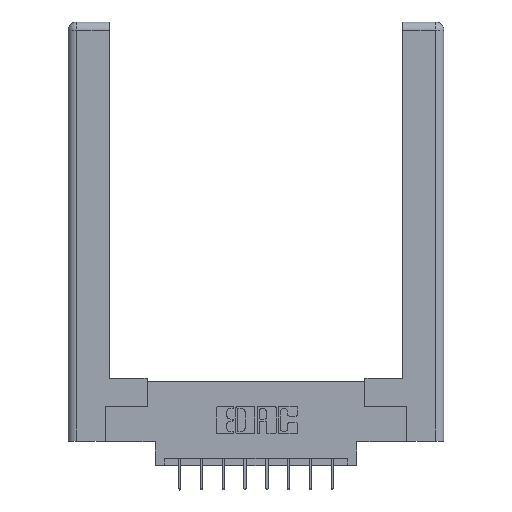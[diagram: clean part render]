
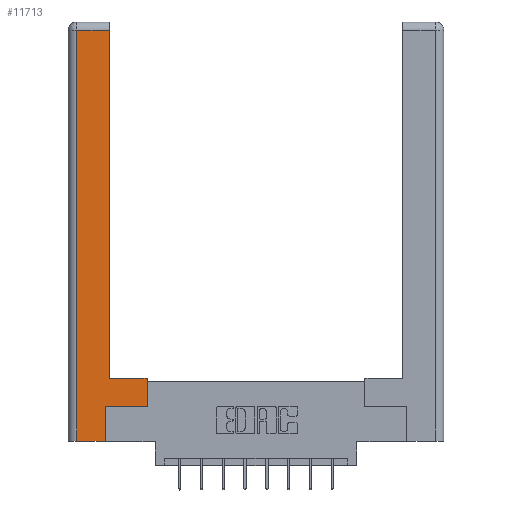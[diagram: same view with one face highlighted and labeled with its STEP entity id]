
A CAD part, top view. The second image highlights one B-rep face of the part: STEP entity #11713.
In plain terms, the highlighted planar face has unit normal (0, 0, 1).
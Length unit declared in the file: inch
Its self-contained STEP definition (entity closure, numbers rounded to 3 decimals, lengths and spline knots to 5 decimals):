
#439 = VERTEX_POINT ( 'NONE', #5067 ) ;
#670 = AXIS2_PLACEMENT_3D ( 'NONE', #10970, #13184, #11152 ) ;
#1038 = CARTESIAN_POINT ( 'NONE',  ( 0.265, 0.245, 0. ) ) ;
#1126 = DIRECTION ( 'NONE',  ( 0., 1., 0. ) ) ;
#1626 = LINE ( 'NONE', #8854, #5019 ) ;
#1725 = ORIENTED_EDGE ( 'NONE', *, *, #13055, .T. ) ;
#1729 = ORIENTED_EDGE ( 'NONE', *, *, #2698, .T. ) ;
#1742 = DIRECTION ( 'NONE',  ( -1., 0., 0. ) ) ;
#1770 = VECTOR ( 'NONE', #6748, 39.37008 ) ;
#1803 = CARTESIAN_POINT ( 'NONE',  ( 0.265, 0., 0. ) ) ;
#1998 = DIRECTION ( 'NONE',  ( 1., 0., 0. ) ) ;
#2093 = EDGE_CURVE ( 'NONE', #8377, #6248, #12899, .T. ) ;
#2221 = VERTEX_POINT ( 'NONE', #5303 ) ;
#2244 = CARTESIAN_POINT ( 'NONE',  ( 0.295, 0.45, 0. ) ) ;
#2698 = EDGE_CURVE ( 'NONE', #7606, #6331, #7299, .T. ) ;
#3141 = EDGE_CURVE ( 'NONE', #6331, #7619, #6506, .T. ) ;
#3749 = ORIENTED_EDGE ( 'NONE', *, *, #11745, .T. ) ;
#4716 = CARTESIAN_POINT ( 'NONE',  ( 0.295, 3., 0. ) ) ;
#4830 = CARTESIAN_POINT ( 'NONE',  ( 0.565, 0.245, 0. ) ) ;
#5000 = CARTESIAN_POINT ( 'NONE',  ( 0.0615, 0., 0. ) ) ;
#5019 = VECTOR ( 'NONE', #1742, 39.37008 ) ;
#5067 = CARTESIAN_POINT ( 'NONE',  ( 0.565, 0.45, 0. ) ) ;
#5303 = CARTESIAN_POINT ( 'NONE',  ( 0.295, 2.94, 0. ) ) ;
#5574 = ORIENTED_EDGE ( 'NONE', *, *, #13428, .T. ) ;
#5677 = FACE_OUTER_BOUND ( 'NONE', #7640, .T. ) ;
#6065 = CARTESIAN_POINT ( 'NONE',  ( 0.565, 0.245, 0. ) ) ;
#6248 = VERTEX_POINT ( 'NONE', #4830 ) ;
#6330 = DIRECTION ( 'NONE',  ( 0., 1., 0. ) ) ;
#6331 = VERTEX_POINT ( 'NONE', #5000 ) ;
#6367 = ORIENTED_EDGE ( 'NONE', *, *, #8719, .T. ) ;
#6506 = LINE ( 'NONE', #10055, #7625 ) ;
#6741 = ORIENTED_EDGE ( 'NONE', *, *, #3141, .T. ) ;
#6748 = DIRECTION ( 'NONE',  ( 0., 1., 0. ) ) ;
#7018 = DIRECTION ( 'NONE',  ( -1., 0., 0. ) ) ;
#7156 = EDGE_CURVE ( 'NONE', #6248, #439, #10647, .T. ) ;
#7299 = LINE ( 'NONE', #7447, #9768 ) ;
#7447 = CARTESIAN_POINT ( 'NONE',  ( 0.0615, 0., 0. ) ) ;
#7606 = VERTEX_POINT ( 'NONE', #7853 ) ;
#7619 = VERTEX_POINT ( 'NONE', #1803 ) ;
#7625 = VECTOR ( 'NONE', #9105, 39.37008 ) ;
#7640 = EDGE_LOOP ( 'NONE', ( #1725, #3749, #1729, #6741, #5574, #8189, #9995, #6367 ) ) ;
#7853 = CARTESIAN_POINT ( 'NONE',  ( 0.0615, 2.94, 0. ) ) ;
#7855 = VECTOR ( 'NONE', #6330, 39.37008 ) ;
#8028 = CARTESIAN_POINT ( 'NONE',  ( 0.295, 0.45, 0. ) ) ;
#8189 = ORIENTED_EDGE ( 'NONE', *, *, #2093, .T. ) ;
#8377 = VERTEX_POINT ( 'NONE', #1038 ) ;
#8391 = LINE ( 'NONE', #11454, #10867 ) ;
#8513 = CARTESIAN_POINT ( 'NONE',  ( 0.565, 0.45, 0. ) ) ;
#8719 = EDGE_CURVE ( 'NONE', #439, #9327, #10819, .T. ) ;
#8854 = CARTESIAN_POINT ( 'NONE',  ( 0.0615, 2.94, 0. ) ) ;
#8966 = VECTOR ( 'NONE', #1998, 39.37008 ) ;
#9105 = DIRECTION ( 'NONE',  ( 1., 0., 0. ) ) ;
#9175 = VECTOR ( 'NONE', #7018, 39.37008 ) ;
#9327 = VERTEX_POINT ( 'NONE', #2244 ) ;
#9389 = DIRECTION ( 'NONE',  ( 0., -1., 0. ) ) ;
#9768 = VECTOR ( 'NONE', #9389, 39.37008 ) ;
#9995 = ORIENTED_EDGE ( 'NONE', *, *, #7156, .T. ) ;
#10055 = CARTESIAN_POINT ( 'NONE',  ( 0.265, 0., 0. ) ) ;
#10071 = PLANE ( 'NONE',  #670 ) ;
#10647 = LINE ( 'NONE', #8513, #7855 ) ;
#10819 = LINE ( 'NONE', #8028, #9175 ) ;
#10867 = VECTOR ( 'NONE', #1126, 39.37008 ) ;
#10970 = CARTESIAN_POINT ( 'NONE',  ( 0., 0., 0. ) ) ;
#11152 = DIRECTION ( 'NONE',  ( -1., 0., 0. ) ) ;
#11454 = CARTESIAN_POINT ( 'NONE',  ( 0.265, 0.245, 0. ) ) ;
#11706 = LINE ( 'NONE', #4716, #1770 ) ;
#11713 = ADVANCED_FACE ( 'NONE', ( #5677 ), #10071, .F. ) ;
#11745 = EDGE_CURVE ( 'NONE', #2221, #7606, #1626, .T. ) ;
#12899 = LINE ( 'NONE', #6065, #8966 ) ;
#13055 = EDGE_CURVE ( 'NONE', #9327, #2221, #11706, .T. ) ;
#13184 = DIRECTION ( 'NONE',  ( 0., 0., -1. ) ) ;
#13428 = EDGE_CURVE ( 'NONE', #7619, #8377, #8391, .T. ) ;
